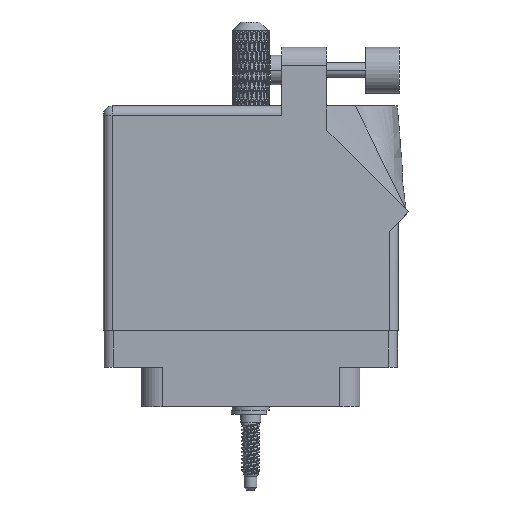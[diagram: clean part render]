
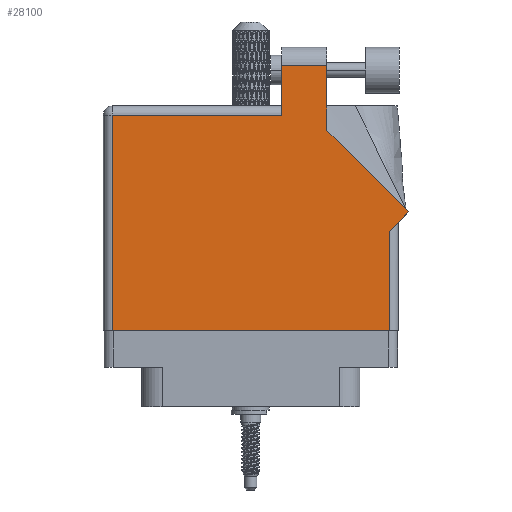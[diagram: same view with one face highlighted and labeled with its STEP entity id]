
A CAD part, front view. The second image highlights one B-rep face of the part: STEP entity #28100.
In plain terms, the highlighted face is planar.
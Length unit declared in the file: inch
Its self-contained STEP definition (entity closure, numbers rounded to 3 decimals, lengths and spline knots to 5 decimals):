
#131 = ORIENTED_EDGE ( 'NONE', *, *, #10519, .T. ) ;
#1556 = VERTEX_POINT ( 'NONE', #2015 ) ;
#1845 = CARTESIAN_POINT ( 'NONE',  ( 0.212, 1.705, 0.455 ) ) ;
#2015 = CARTESIAN_POINT ( 'NONE',  ( 0.519, 1.705, 0.455 ) ) ;
#2196 = DIRECTION ( 'NONE',  ( -1., 0., 0. ) ) ;
#2811 = EDGE_CURVE ( 'NONE', #21572, #10255, #45838, .T. ) ;
#3187 = LINE ( 'NONE', #59803, #97726 ) ;
#6685 = CARTESIAN_POINT ( 'NONE',  ( -1.005, 1.43, 0.455 ) ) ;
#7326 = VECTOR ( 'NONE', #83549, 39.37008 ) ;
#7687 = LINE ( 'NONE', #30116, #49699 ) ;
#8595 = ORIENTED_EDGE ( 'NONE', *, *, #42319, .T. ) ;
#10255 = VERTEX_POINT ( 'NONE', #87920 ) ;
#10519 = EDGE_CURVE ( 'NONE', #48253, #83290, #83879, .T. ) ;
#10957 = DIRECTION ( 'NONE',  ( 0., 1., 0. ) ) ;
#13054 = EDGE_CURVE ( 'NONE', #83290, #1556, #3187, .T. ) ;
#14324 = VECTOR ( 'NONE', #64961, 39.37008 ) ;
#18528 = VECTOR ( 'NONE', #19163, 39.37008 ) ;
#19163 = DIRECTION ( 'NONE',  ( 0., -1., 0. ) ) ;
#21572 = VERTEX_POINT ( 'NONE', #94877 ) ;
#21800 = ORIENTED_EDGE ( 'NONE', *, *, #2811, .T. ) ;
#24232 = VECTOR ( 'NONE', #35934, 39.37008 ) ;
#25341 = CARTESIAN_POINT ( 'NONE',  ( -1.005, 1.368, 0.455 ) ) ;
#26030 = EDGE_LOOP ( 'NONE', ( #84251, #34463, #21800, #8595, #42531, #62421, #80903, #81839, #131 ) ) ;
#26247 = EDGE_CURVE ( 'NONE', #36496, #94326, #31263, .T. ) ;
#27966 = LINE ( 'NONE', #25341, #68848 ) ;
#28100 = ADVANCED_FACE ( 'NONE', ( #65346 ), #56578, .F. ) ;
#29091 = EDGE_CURVE ( 'NONE', #94326, #63267, #57661, .T. ) ;
#30116 = CARTESIAN_POINT ( 'NONE',  ( 1.005, 0.637, 0.455 ) ) ;
#31263 = LINE ( 'NONE', #68001, #18528 ) ;
#34463 = ORIENTED_EDGE ( 'NONE', *, *, #35436, .T. ) ;
#34599 = CARTESIAN_POINT ( 'NONE',  ( 1.07571, 0.70771, 0.455 ) ) ;
#35436 = EDGE_CURVE ( 'NONE', #1556, #21572, #58746, .T. ) ;
#35934 = DIRECTION ( 'NONE',  ( 0., -1., 0. ) ) ;
#36225 = LINE ( 'NONE', #47250, #81077 ) ;
#36496 = VERTEX_POINT ( 'NONE', #49342 ) ;
#39743 = DIRECTION ( 'NONE',  ( 0., 1., 0. ) ) ;
#40135 = DIRECTION ( 'NONE',  ( -1., 0., 0. ) ) ;
#42319 = EDGE_CURVE ( 'NONE', #10255, #36496, #27966, .T. ) ;
#42531 = ORIENTED_EDGE ( 'NONE', *, *, #26247, .T. ) ;
#45838 = LINE ( 'NONE', #93126, #24232 ) ;
#47250 = CARTESIAN_POINT ( 'NONE',  ( 0.943, 0.637, 0.455 ) ) ;
#48253 = VERTEX_POINT ( 'NONE', #65287 ) ;
#49342 = CARTESIAN_POINT ( 'NONE',  ( -0.943, 1.368, 0.455 ) ) ;
#49699 = VECTOR ( 'NONE', #70448, 39.37008 ) ;
#49775 = VECTOR ( 'NONE', #2196, 39.37008 ) ;
#53236 = CARTESIAN_POINT ( 'NONE',  ( 0.943, -0.1, 0.455 ) ) ;
#53661 = VERTEX_POINT ( 'NONE', #79085 ) ;
#56578 = PLANE ( 'NONE',  #87706 ) ;
#57661 = LINE ( 'NONE', #72487, #14324 ) ;
#58746 = LINE ( 'NONE', #1845, #49775 ) ;
#59803 = CARTESIAN_POINT ( 'NONE',  ( 0.519, 1.26442, 0.455 ) ) ;
#60948 = EDGE_CURVE ( 'NONE', #53661, #48253, #7687, .T. ) ;
#62421 = ORIENTED_EDGE ( 'NONE', *, *, #29091, .T. ) ;
#63267 = VERTEX_POINT ( 'NONE', #53236 ) ;
#64961 = DIRECTION ( 'NONE',  ( 1., 0., 0. ) ) ;
#65287 = CARTESIAN_POINT ( 'NONE',  ( 1.07571, 0.70771, 0.455 ) ) ;
#65346 = FACE_OUTER_BOUND ( 'NONE', #26030, .T. ) ;
#68001 = CARTESIAN_POINT ( 'NONE',  ( -0.943, -0.1, 0.455 ) ) ;
#68848 = VECTOR ( 'NONE', #90995, 39.37008 ) ;
#70448 = DIRECTION ( 'NONE',  ( 0.707, 0.707, 0. ) ) ;
#72487 = CARTESIAN_POINT ( 'NONE',  ( -1.005, -0.1, 0.455 ) ) ;
#73764 = CARTESIAN_POINT ( 'NONE',  ( 0.519, 1.26442, 0.455 ) ) ;
#79085 = CARTESIAN_POINT ( 'NONE',  ( 0.943, 0.575, 0.455 ) ) ;
#79816 = CARTESIAN_POINT ( 'NONE',  ( -0.943, -0.1, 0.455 ) ) ;
#80903 = ORIENTED_EDGE ( 'NONE', *, *, #84764, .T. ) ;
#81077 = VECTOR ( 'NONE', #39743, 39.37008 ) ;
#81839 = ORIENTED_EDGE ( 'NONE', *, *, #60948, .T. ) ;
#83290 = VERTEX_POINT ( 'NONE', #73764 ) ;
#83549 = DIRECTION ( 'NONE',  ( -0.707, 0.707, 0. ) ) ;
#83879 = LINE ( 'NONE', #34599, #7326 ) ;
#84251 = ORIENTED_EDGE ( 'NONE', *, *, #13054, .T. ) ;
#84764 = EDGE_CURVE ( 'NONE', #63267, #53661, #36225, .T. ) ;
#87706 = AXIS2_PLACEMENT_3D ( 'NONE', #6685, #105932, #40135 ) ;
#87920 = CARTESIAN_POINT ( 'NONE',  ( 0.212, 1.368, 0.455 ) ) ;
#90995 = DIRECTION ( 'NONE',  ( -1., 0., 0. ) ) ;
#93126 = CARTESIAN_POINT ( 'NONE',  ( 0.212, 1.43, 0.455 ) ) ;
#94326 = VERTEX_POINT ( 'NONE', #79816 ) ;
#94877 = CARTESIAN_POINT ( 'NONE',  ( 0.212, 1.705, 0.455 ) ) ;
#97726 = VECTOR ( 'NONE', #10957, 39.37008 ) ;
#105932 = DIRECTION ( 'NONE',  ( 0., 0., -1. ) ) ;
